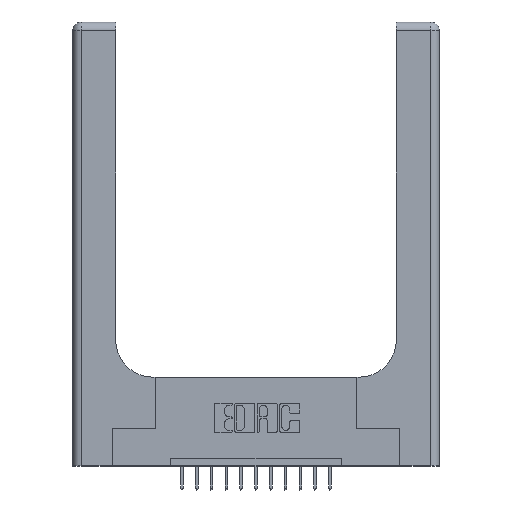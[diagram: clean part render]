
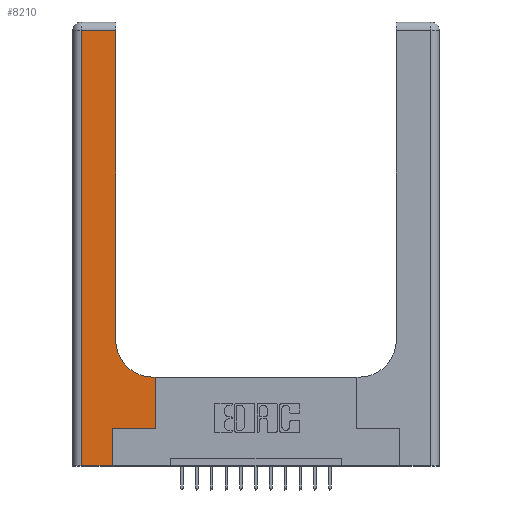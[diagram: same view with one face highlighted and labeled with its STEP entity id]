
A CAD part, top view. The second image highlights one B-rep face of the part: STEP entity #8210.
In plain terms, the highlighted planar face has unit normal (0, 0, 1).
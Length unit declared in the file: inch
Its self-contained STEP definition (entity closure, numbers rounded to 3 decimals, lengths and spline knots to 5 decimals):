
#366 = DIRECTION ( 'NONE',  ( 1., 0., 0. ) ) ;
#483 = EDGE_CURVE ( 'NONE', #5596, #16261, #14444, .T. ) ;
#544 = CARTESIAN_POINT ( 'NONE',  ( 0.06, 2.94, 0.37 ) ) ;
#830 = CARTESIAN_POINT ( 'NONE',  ( 0.06, 3., 0.37 ) ) ;
#836 = VECTOR ( 'NONE', #6874, 39.37008 ) ;
#964 = DIRECTION ( 'NONE',  ( -1., 0., 0. ) ) ;
#971 = EDGE_CURVE ( 'NONE', #17427, #9732, #15929, .T. ) ;
#1114 = VECTOR ( 'NONE', #964, 39.37008 ) ;
#1202 = CARTESIAN_POINT ( 'NONE',  ( 0.269, 0., 0.37 ) ) ;
#1494 = ORIENTED_EDGE ( 'NONE', *, *, #7806, .T. ) ;
#1744 = CARTESIAN_POINT ( 'NONE',  ( 0.5585, 0.25, 0.37 ) ) ;
#1893 = DIRECTION ( 'NONE',  ( 1., 0., 0. ) ) ;
#2176 = VECTOR ( 'NONE', #10492, 39.37008 ) ;
#2804 = ORIENTED_EDGE ( 'NONE', *, *, #971, .T. ) ;
#2894 = ORIENTED_EDGE ( 'NONE', *, *, #13469, .T. ) ;
#2993 = CARTESIAN_POINT ( 'NONE',  ( 0.269, 0.25, 0.37 ) ) ;
#3112 = VECTOR ( 'NONE', #16402, 39.37008 ) ;
#3131 = CARTESIAN_POINT ( 'NONE',  ( 0., 0., 0.37 ) ) ;
#3237 = CIRCLE ( 'NONE', #11660, 0.25 ) ;
#3283 = DIRECTION ( 'NONE',  ( 0., 1., 0. ) ) ;
#3319 = CARTESIAN_POINT ( 'NONE',  ( 0.5415, 0.85, 0.37 ) ) ;
#3391 = EDGE_CURVE ( 'NONE', #9732, #4835, #12230, .T. ) ;
#3431 = LINE ( 'NONE', #13245, #2176 ) ;
#4243 = EDGE_CURVE ( 'NONE', #13108, #5596, #12192, .T. ) ;
#4303 = PLANE ( 'NONE',  #12080 ) ;
#4803 = DIRECTION ( 'NONE',  ( 0., 0., -1. ) ) ;
#4835 = VERTEX_POINT ( 'NONE', #8225 ) ;
#4914 = EDGE_LOOP ( 'NONE', ( #16467, #15658, #8529, #1494, #2894, #17049, #2804, #11721, #14987 ) ) ;
#5157 = EDGE_CURVE ( 'NONE', #4835, #13108, #3237, .T. ) ;
#5225 = DIRECTION ( 'NONE',  ( 0., -1., 0. ) ) ;
#5301 = LINE ( 'NONE', #2993, #836 ) ;
#5596 = VERTEX_POINT ( 'NONE', #6713 ) ;
#6091 = VECTOR ( 'NONE', #3283, 39.37008 ) ;
#6236 = VERTEX_POINT ( 'NONE', #10872 ) ;
#6713 = CARTESIAN_POINT ( 'NONE',  ( 0.2915, 2.94, 0.37 ) ) ;
#6804 = CARTESIAN_POINT ( 'NONE',  ( 0., 2.94, 0.37 ) ) ;
#6874 = DIRECTION ( 'NONE',  ( 1., 0., 0. ) ) ;
#7806 = EDGE_CURVE ( 'NONE', #6236, #14250, #16689, .T. ) ;
#8053 = VECTOR ( 'NONE', #5225, 39.37008 ) ;
#8210 = ADVANCED_FACE ( 'NONE', ( #10291 ), #4303, .F. ) ;
#8225 = CARTESIAN_POINT ( 'NONE',  ( 0.5415, 0.6, 0.37 ) ) ;
#8529 = ORIENTED_EDGE ( 'NONE', *, *, #15906, .T. ) ;
#8558 = CARTESIAN_POINT ( 'NONE',  ( 0., 3., 0.37 ) ) ;
#9235 = VECTOR ( 'NONE', #14875, 39.37008 ) ;
#9355 = CARTESIAN_POINT ( 'NONE',  ( 0.2915, 3., 0.37 ) ) ;
#9732 = VERTEX_POINT ( 'NONE', #14928 ) ;
#9964 = LINE ( 'NONE', #830, #8053 ) ;
#10291 = FACE_OUTER_BOUND ( 'NONE', #4914, .T. ) ;
#10492 = DIRECTION ( 'NONE',  ( 0., 1., 0. ) ) ;
#10571 = CARTESIAN_POINT ( 'NONE',  ( 0.2915, 0.85, 0.37 ) ) ;
#10872 = CARTESIAN_POINT ( 'NONE',  ( 0.06, 0., 0.37 ) ) ;
#11660 = AXIS2_PLACEMENT_3D ( 'NONE', #3319, #4803, #1893 ) ;
#11721 = ORIENTED_EDGE ( 'NONE', *, *, #3391, .T. ) ;
#12080 = AXIS2_PLACEMENT_3D ( 'NONE', #8558, #12446, #12143 ) ;
#12143 = DIRECTION ( 'NONE',  ( -1., 0., 0. ) ) ;
#12192 = LINE ( 'NONE', #9355, #9235 ) ;
#12230 = LINE ( 'NONE', #17321, #1114 ) ;
#12446 = DIRECTION ( 'NONE',  ( 0., 0., -1. ) ) ;
#13108 = VERTEX_POINT ( 'NONE', #10571 ) ;
#13245 = CARTESIAN_POINT ( 'NONE',  ( 0.269, 0., 0.37 ) ) ;
#13299 = VECTOR ( 'NONE', #366, 39.37008 ) ;
#13469 = EDGE_CURVE ( 'NONE', #14250, #16597, #3431, .T. ) ;
#14250 = VERTEX_POINT ( 'NONE', #1202 ) ;
#14283 = EDGE_CURVE ( 'NONE', #16597, #17427, #5301, .T. ) ;
#14444 = LINE ( 'NONE', #6804, #3112 ) ;
#14875 = DIRECTION ( 'NONE',  ( 0., 1., 0. ) ) ;
#14928 = CARTESIAN_POINT ( 'NONE',  ( 0.5585, 0.6, 0.37 ) ) ;
#14987 = ORIENTED_EDGE ( 'NONE', *, *, #5157, .T. ) ;
#15248 = CARTESIAN_POINT ( 'NONE',  ( 0.269, 0.25, 0.37 ) ) ;
#15658 = ORIENTED_EDGE ( 'NONE', *, *, #483, .T. ) ;
#15906 = EDGE_CURVE ( 'NONE', #16261, #6236, #9964, .T. ) ;
#15929 = LINE ( 'NONE', #1744, #6091 ) ;
#16261 = VERTEX_POINT ( 'NONE', #544 ) ;
#16402 = DIRECTION ( 'NONE',  ( -1., 0., 0. ) ) ;
#16467 = ORIENTED_EDGE ( 'NONE', *, *, #4243, .T. ) ;
#16597 = VERTEX_POINT ( 'NONE', #15248 ) ;
#16689 = LINE ( 'NONE', #3131, #13299 ) ;
#16831 = CARTESIAN_POINT ( 'NONE',  ( 0.5585, 0.25, 0.37 ) ) ;
#17049 = ORIENTED_EDGE ( 'NONE', *, *, #14283, .T. ) ;
#17321 = CARTESIAN_POINT ( 'NONE',  ( 0.2915, 0.6, 0.37 ) ) ;
#17427 = VERTEX_POINT ( 'NONE', #16831 ) ;
